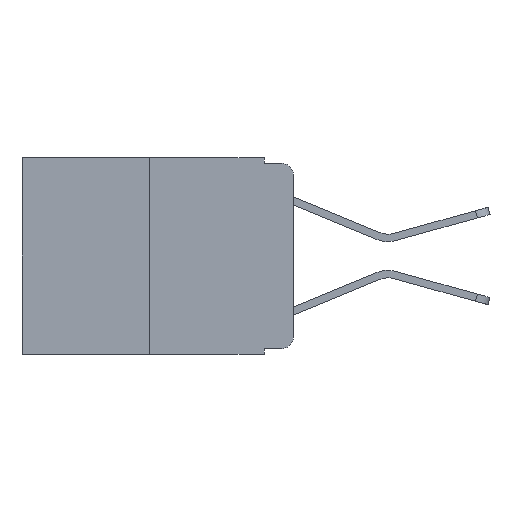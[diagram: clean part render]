
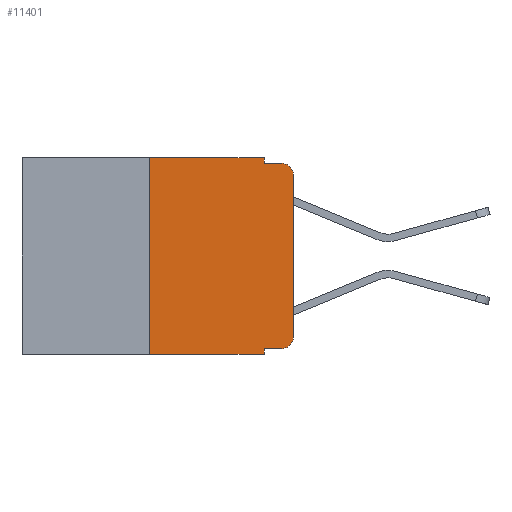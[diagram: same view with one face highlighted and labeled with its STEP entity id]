
A CAD part, left-side view. The second image highlights one B-rep face of the part: STEP entity #11401.
In plain terms, the highlighted planar face has unit normal (-1, 0, 0).
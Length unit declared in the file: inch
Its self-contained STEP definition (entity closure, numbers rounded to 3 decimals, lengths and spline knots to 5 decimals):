
#2 = EDGE_CURVE ( 'NONE', #9613, #8761, #8040, .T. ) ;
#369 = VERTEX_POINT ( 'NONE', #686 ) ;
#483 = LINE ( 'NONE', #13043, #9861 ) ;
#555 = EDGE_CURVE ( 'NONE', #9613, #2834, #12808, .T. ) ;
#686 = CARTESIAN_POINT ( 'NONE',  ( 0., 0.051, 0. ) ) ;
#709 = EDGE_LOOP ( 'NONE', ( #11154, #6874, #8409, #2411, #15053, #3185, #6866, #5758, #13654, #13982 ) ) ;
#1030 = CIRCLE ( 'NONE', #11220, 0.02 ) ;
#1098 = VERTEX_POINT ( 'NONE', #11355 ) ;
#1756 = CARTESIAN_POINT ( 'NONE',  ( 0., 0.25, 0. ) ) ;
#2340 = LINE ( 'NONE', #3606, #5408 ) ;
#2411 = ORIENTED_EDGE ( 'NONE', *, *, #6323, .F. ) ;
#2453 = CARTESIAN_POINT ( 'NONE',  ( 0., 0., 0. ) ) ;
#2726 = DIRECTION ( 'NONE',  ( 0., -1., 0. ) ) ;
#2834 = VERTEX_POINT ( 'NONE', #12400 ) ;
#3009 = EDGE_CURVE ( 'NONE', #5548, #8761, #483, .T. ) ;
#3098 = CARTESIAN_POINT ( 'NONE',  ( 0., 0.02, -0.01 ) ) ;
#3185 = ORIENTED_EDGE ( 'NONE', *, *, #9601, .F. ) ;
#3606 = CARTESIAN_POINT ( 'NONE',  ( 0., 0.473, 0. ) ) ;
#3634 = EDGE_CURVE ( 'NONE', #12336, #9434, #13436, .T. ) ;
#3995 = CIRCLE ( 'NONE', #13019, 0.02 ) ;
#4040 = DIRECTION ( 'NONE',  ( 0., -1., 0. ) ) ;
#4413 = DIRECTION ( 'NONE',  ( 0., 0., 1. ) ) ;
#4475 = CARTESIAN_POINT ( 'NONE',  ( 0., 0.051, -0.333 ) ) ;
#4626 = EDGE_CURVE ( 'NONE', #9434, #11338, #1030, .T. ) ;
#4845 = CARTESIAN_POINT ( 'NONE',  ( 0., 0.25, 0. ) ) ;
#5107 = EDGE_CURVE ( 'NONE', #13195, #369, #2340, .T. ) ;
#5254 = VECTOR ( 'NONE', #15141, 39.37008 ) ;
#5408 = VECTOR ( 'NONE', #6109, 39.37008 ) ;
#5548 = VERTEX_POINT ( 'NONE', #6234 ) ;
#5598 = DIRECTION ( 'NONE',  ( -1., 0., 0. ) ) ;
#5758 = ORIENTED_EDGE ( 'NONE', *, *, #2, .F. ) ;
#5765 = DIRECTION ( 'NONE',  ( 1., 0., 0. ) ) ;
#5789 = DIRECTION ( 'NONE',  ( -1., 0., 0. ) ) ;
#6081 = VECTOR ( 'NONE', #14853, 39.37008 ) ;
#6109 = DIRECTION ( 'NONE',  ( 0., -1., 0. ) ) ;
#6234 = CARTESIAN_POINT ( 'NONE',  ( 0., 0.25, -0.343 ) ) ;
#6323 = EDGE_CURVE ( 'NONE', #369, #1098, #8687, .T. ) ;
#6475 = LINE ( 'NONE', #1756, #15164 ) ;
#6520 = LINE ( 'NONE', #9734, #14864 ) ;
#6866 = ORIENTED_EDGE ( 'NONE', *, *, #3009, .T. ) ;
#6874 = ORIENTED_EDGE ( 'NONE', *, *, #4626, .T. ) ;
#7607 = CARTESIAN_POINT ( 'NONE',  ( 0., 0., -0.03 ) ) ;
#7722 = EDGE_CURVE ( 'NONE', #1098, #11338, #6520, .T. ) ;
#8021 = PLANE ( 'NONE',  #12839 ) ;
#8040 = LINE ( 'NONE', #14195, #5254 ) ;
#8353 = CARTESIAN_POINT ( 'NONE',  ( 0., 0.051, 0. ) ) ;
#8409 = ORIENTED_EDGE ( 'NONE', *, *, #7722, .F. ) ;
#8687 = LINE ( 'NONE', #8353, #6081 ) ;
#8761 = VERTEX_POINT ( 'NONE', #9862 ) ;
#9096 = DIRECTION ( 'NONE',  ( 0., 0., -1. ) ) ;
#9434 = VERTEX_POINT ( 'NONE', #7607 ) ;
#9514 = DIRECTION ( 'NONE',  ( 0., 0., 1. ) ) ;
#9541 = EDGE_CURVE ( 'NONE', #2834, #12336, #3995, .T. ) ;
#9601 = EDGE_CURVE ( 'NONE', #5548, #13195, #6475, .T. ) ;
#9613 = VERTEX_POINT ( 'NONE', #4475 ) ;
#9734 = CARTESIAN_POINT ( 'NONE',  ( 0., 0.051, -0.01 ) ) ;
#9861 = VECTOR ( 'NONE', #4040, 39.37008 ) ;
#9862 = CARTESIAN_POINT ( 'NONE',  ( 0., 0.051, -0.343 ) ) ;
#9899 = VECTOR ( 'NONE', #11102, 39.37008 ) ;
#10188 = CARTESIAN_POINT ( 'NONE',  ( 0., 0.051, -0.333 ) ) ;
#10235 = CARTESIAN_POINT ( 'NONE',  ( 0., 0., -0.313 ) ) ;
#10880 = VECTOR ( 'NONE', #9514, 39.37008 ) ;
#11102 = DIRECTION ( 'NONE',  ( 0., -1., 0. ) ) ;
#11154 = ORIENTED_EDGE ( 'NONE', *, *, #3634, .T. ) ;
#11220 = AXIS2_PLACEMENT_3D ( 'NONE', #12361, #5789, #13460 ) ;
#11338 = VERTEX_POINT ( 'NONE', #3098 ) ;
#11355 = CARTESIAN_POINT ( 'NONE',  ( 0., 0.051, -0.01 ) ) ;
#11401 = ADVANCED_FACE ( 'NONE', ( #14468 ), #8021, .F. ) ;
#12189 = CARTESIAN_POINT ( 'NONE',  ( 0., 0.02, -0.313 ) ) ;
#12336 = VERTEX_POINT ( 'NONE', #10235 ) ;
#12361 = CARTESIAN_POINT ( 'NONE',  ( 0., 0.02, -0.03 ) ) ;
#12400 = CARTESIAN_POINT ( 'NONE',  ( 0., 0.02, -0.333 ) ) ;
#12808 = LINE ( 'NONE', #10188, #9899 ) ;
#12839 = AXIS2_PLACEMENT_3D ( 'NONE', #13441, #5765, #9096 ) ;
#13019 = AXIS2_PLACEMENT_3D ( 'NONE', #12189, #5598, #13286 ) ;
#13043 = CARTESIAN_POINT ( 'NONE',  ( 0., 0.473, -0.343 ) ) ;
#13195 = VERTEX_POINT ( 'NONE', #4845 ) ;
#13286 = DIRECTION ( 'NONE',  ( 0., 0., -1. ) ) ;
#13436 = LINE ( 'NONE', #2453, #10880 ) ;
#13441 = CARTESIAN_POINT ( 'NONE',  ( 0., 0.473, 0. ) ) ;
#13460 = DIRECTION ( 'NONE',  ( 0., 0., -1. ) ) ;
#13654 = ORIENTED_EDGE ( 'NONE', *, *, #555, .T. ) ;
#13982 = ORIENTED_EDGE ( 'NONE', *, *, #9541, .T. ) ;
#14195 = CARTESIAN_POINT ( 'NONE',  ( 0., 0.051, 0. ) ) ;
#14468 = FACE_OUTER_BOUND ( 'NONE', #709, .T. ) ;
#14853 = DIRECTION ( 'NONE',  ( 0., 0., -1. ) ) ;
#14864 = VECTOR ( 'NONE', #2726, 39.37008 ) ;
#15053 = ORIENTED_EDGE ( 'NONE', *, *, #5107, .F. ) ;
#15141 = DIRECTION ( 'NONE',  ( 0., 0., -1. ) ) ;
#15164 = VECTOR ( 'NONE', #4413, 39.37008 ) ;
